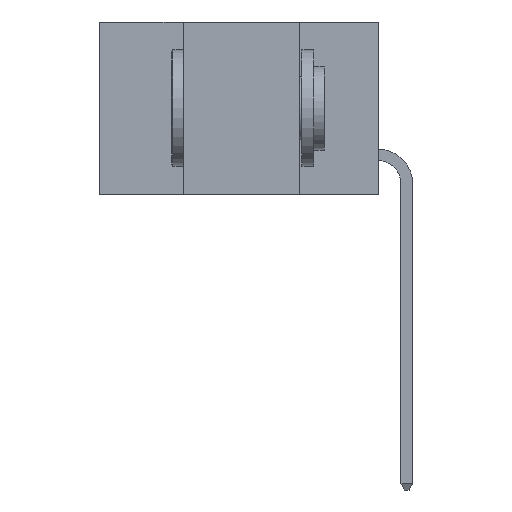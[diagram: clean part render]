
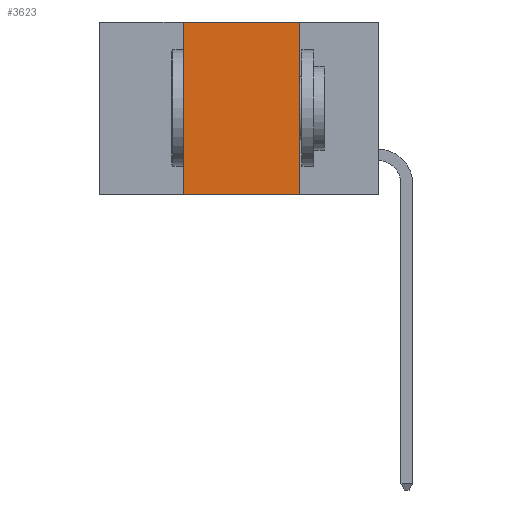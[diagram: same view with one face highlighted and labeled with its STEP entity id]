
A CAD part, left-side view. The second image highlights one B-rep face of the part: STEP entity #3623.
In plain terms, the highlighted planar face has unit normal (-1, 0, 0).
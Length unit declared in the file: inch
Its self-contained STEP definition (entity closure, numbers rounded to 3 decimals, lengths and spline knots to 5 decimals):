
#874 = CARTESIAN_POINT ( 'NONE',  ( 0., 0.17, -0.37 ) ) ;
#1022 = CARTESIAN_POINT ( 'NONE',  ( 0., 0.6, 0. ) ) ;
#1046 = DIRECTION ( 'NONE',  ( 0., -1., 0. ) ) ;
#2793 = VERTEX_POINT ( 'NONE', #19955 ) ;
#3623 = ADVANCED_FACE ( 'NONE', ( #9241 ), #10906, .F. ) ;
#3770 = DIRECTION ( 'NONE',  ( 0., -1., 0. ) ) ;
#4501 = CARTESIAN_POINT ( 'NONE',  ( 0., 0.6, -0.37 ) ) ;
#9107 = VERTEX_POINT ( 'NONE', #16829 ) ;
#9241 = FACE_OUTER_BOUND ( 'NONE', #18049, .T. ) ;
#9521 = EDGE_CURVE ( 'NONE', #9627, #9107, #16982, .T. ) ;
#9627 = VERTEX_POINT ( 'NONE', #21513 ) ;
#10174 = DIRECTION ( 'NONE',  ( 0., 0., -1. ) ) ;
#10230 = DIRECTION ( 'NONE',  ( 1., 0., 0. ) ) ;
#10310 = CARTESIAN_POINT ( 'NONE',  ( 0., 0.6, 0. ) ) ;
#10906 = PLANE ( 'NONE',  #17912 ) ;
#11382 = VERTEX_POINT ( 'NONE', #17995 ) ;
#12728 = VECTOR ( 'NONE', #3770, 39.37008 ) ;
#13871 = CARTESIAN_POINT ( 'NONE',  ( 0., 0.42, -0.37 ) ) ;
#13893 = DIRECTION ( 'NONE',  ( 0., 0., 1. ) ) ;
#15601 = EDGE_CURVE ( 'NONE', #9627, #2793, #15823, .T. ) ;
#15823 = LINE ( 'NONE', #13871, #22544 ) ;
#16829 = CARTESIAN_POINT ( 'NONE',  ( 0., 0.17, -0.37 ) ) ;
#16839 = EDGE_CURVE ( 'NONE', #2793, #11382, #17645, .T. ) ;
#16982 = LINE ( 'NONE', #4501, #12728 ) ;
#17645 = LINE ( 'NONE', #1022, #21826 ) ;
#17791 = LINE ( 'NONE', #874, #21941 ) ;
#17912 = AXIS2_PLACEMENT_3D ( 'NONE', #10310, #10230, #10174 ) ;
#17995 = CARTESIAN_POINT ( 'NONE',  ( 0., 0.17, 0. ) ) ;
#18049 = EDGE_LOOP ( 'NONE', ( #21725, #22163, #23014, #23432 ) ) ;
#19955 = CARTESIAN_POINT ( 'NONE',  ( 0., 0.42, 0. ) ) ;
#20511 = EDGE_CURVE ( 'NONE', #11382, #9107, #17791, .T. ) ;
#21098 = DIRECTION ( 'NONE',  ( 0., 0., -1. ) ) ;
#21513 = CARTESIAN_POINT ( 'NONE',  ( 0., 0.42, -0.37 ) ) ;
#21725 = ORIENTED_EDGE ( 'NONE', *, *, #20511, .F. ) ;
#21826 = VECTOR ( 'NONE', #1046, 39.37008 ) ;
#21941 = VECTOR ( 'NONE', #21098, 39.37008 ) ;
#22163 = ORIENTED_EDGE ( 'NONE', *, *, #16839, .F. ) ;
#22544 = VECTOR ( 'NONE', #13893, 39.37008 ) ;
#23014 = ORIENTED_EDGE ( 'NONE', *, *, #15601, .F. ) ;
#23432 = ORIENTED_EDGE ( 'NONE', *, *, #9521, .T. ) ;
